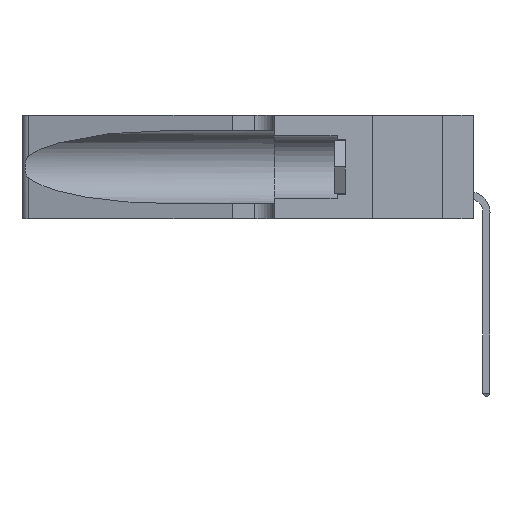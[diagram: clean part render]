
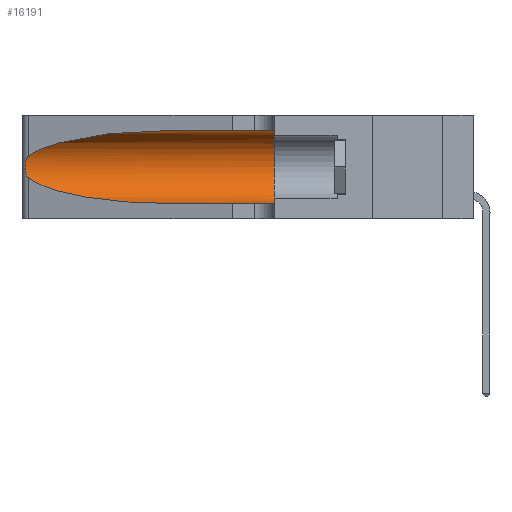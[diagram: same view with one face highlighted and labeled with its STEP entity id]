
A CAD part, left-side view. The second image highlights one B-rep face of the part: STEP entity #16191.
In plain terms, the highlighted cylindrical face has radius 3.308 mm (diameter 6.617 mm), a partial arc.
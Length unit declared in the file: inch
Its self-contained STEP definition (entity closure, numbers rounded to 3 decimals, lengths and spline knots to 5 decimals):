
#150 = VERTEX_POINT ( 'NONE', #843 ) ;
#653 = VERTEX_POINT ( 'NONE', #6501 ) ;
#745 = B_SPLINE_CURVE_WITH_KNOTS ( 'NONE', 3,
 ( #17289, #8688, #10274, #8830, #12127, #12191, #3586, #5343, #17432, #19124, #15380, #17130, #3381, #6819 ),
 .UNSPECIFIED., .F., .F.,
 ( 4, 2, 2, 2, 2, 2, 4 ),
 ( 0., 0.00027, 0.00053, 0.00107, 0.0016, 0.00187, 0.00214 ),
 .UNSPECIFIED. ) ;
#843 = CARTESIAN_POINT ( 'NONE',  ( 0.1305, 0.72297, 0.31525 ) ) ;
#1633 = CARTESIAN_POINT ( 'NONE',  ( 0.1305, 0.35, 0.31525 ) ) ;
#2723 = CARTESIAN_POINT ( 'NONE',  ( 0.25487, 1.22718, 0.14631 ) ) ;
#2830 = ORIENTED_EDGE ( 'NONE', *, *, #17265, .F. ) ;
#3282 = CARTESIAN_POINT ( 'NONE',  ( 0.1305, 0.72297, 0.05475 ) ) ;
#3381 = CARTESIAN_POINT ( 'NONE',  ( 0.25555, 1.22993, 0.14849 ) ) ;
#3586 = CARTESIAN_POINT ( 'NONE',  ( 0.26075, 1.23896, 0.19203 ) ) ;
#3943 = CARTESIAN_POINT ( 'NONE',  ( 0.1305, 0.35, 0.185 ) ) ;
#4028 = CIRCLE ( 'NONE', #14323, 0.13025 ) ;
#4514 =( BOUNDED_CURVE ( )  B_SPLINE_CURVE ( 3, ( #4868, #8597, #6722, #3282 ),
 .UNSPECIFIED., .F., .F. ) 
 B_SPLINE_CURVE_WITH_KNOTS ( ( 4, 4 ),
 ( 3.44316, 4.71239 ),
 .UNSPECIFIED. ) 
 CURVE ( )  GEOMETRIC_REPRESENTATION_ITEM ( )  RATIONAL_B_SPLINE_CURVE ( ( 1., 0.87, 0.87, 1. ) ) 
 REPRESENTATION_ITEM ( '' )  );
#4747 = CARTESIAN_POINT ( 'NONE',  ( 0.1305, 1.61858, 0.05475 ) ) ;
#4868 = CARTESIAN_POINT ( 'NONE',  ( 0.25487, 1.22718, 0.14631 ) ) ;
#4878 = EDGE_CURVE ( 'NONE', #653, #9045, #8433, .T. ) ;
#5343 = CARTESIAN_POINT ( 'NONE',  ( 0.26075, 1.23896, 0.178 ) ) ;
#5452 = DIRECTION ( 'NONE',  ( 0., 0., -1. ) ) ;
#5642 = EDGE_CURVE ( 'NONE', #150, #10348, #14591, .T. ) ;
#6501 = CARTESIAN_POINT ( 'NONE',  ( 0.1305, 0.72297, 0.05475 ) ) ;
#6722 = CARTESIAN_POINT ( 'NONE',  ( 0.18966, 0.96281, 0.05475 ) ) ;
#6819 = CARTESIAN_POINT ( 'NONE',  ( 0.25487, 1.22718, 0.14631 ) ) ;
#6820 = VECTOR ( 'NONE', #20263, 39.37008 ) ;
#7023 = CARTESIAN_POINT ( 'NONE',  ( 0.1305, 1.61858, 0.31525 ) ) ;
#7446 = EDGE_CURVE ( 'NONE', #10348, #16426, #745, .T. ) ;
#7447 = DIRECTION ( 'NONE',  ( 0., 0., 1. ) ) ;
#7451 = VERTEX_POINT ( 'NONE', #1633 ) ;
#8433 = LINE ( 'NONE', #4747, #6820 ) ;
#8597 = CARTESIAN_POINT ( 'NONE',  ( 0.2373, 1.15595, 0.08982 ) ) ;
#8688 = CARTESIAN_POINT ( 'NONE',  ( 0.25555, 1.22994, 0.2215 ) ) ;
#8807 = CARTESIAN_POINT ( 'NONE',  ( 0.1305, 0.72297, 0.31525 ) ) ;
#8830 = CARTESIAN_POINT ( 'NONE',  ( 0.25787, 1.23484, 0.2124 ) ) ;
#9045 = VERTEX_POINT ( 'NONE', #18593 ) ;
#9908 = EDGE_LOOP ( 'NONE', ( #13677, #14777, #13236, #13305, #10698, #2830 ) ) ;
#10274 = CARTESIAN_POINT ( 'NONE',  ( 0.25639, 1.23184, 0.21858 ) ) ;
#10318 = CARTESIAN_POINT ( 'NONE',  ( 0.18966, 0.96281, 0.31525 ) ) ;
#10348 = VERTEX_POINT ( 'NONE', #16599 ) ;
#10531 = CARTESIAN_POINT ( 'NONE',  ( 0.25487, 1.22718, 0.22369 ) ) ;
#10698 = ORIENTED_EDGE ( 'NONE', *, *, #10965, .F. ) ;
#10965 = EDGE_CURVE ( 'NONE', #7451, #9045, #4028, .T. ) ;
#12127 = CARTESIAN_POINT ( 'NONE',  ( 0.25854, 1.2359, 0.20912 ) ) ;
#12191 = CARTESIAN_POINT ( 'NONE',  ( 0.26018, 1.23835, 0.19895 ) ) ;
#13236 = ORIENTED_EDGE ( 'NONE', *, *, #14409, .T. ) ;
#13305 = ORIENTED_EDGE ( 'NONE', *, *, #4878, .T. ) ;
#13535 = AXIS2_PLACEMENT_3D ( 'NONE', #19157, #13953, #5452 ) ;
#13677 = ORIENTED_EDGE ( 'NONE', *, *, #5642, .T. ) ;
#13953 = DIRECTION ( 'NONE',  ( 0., -1., 0. ) ) ;
#14323 = AXIS2_PLACEMENT_3D ( 'NONE', #3943, #20861, #7447 ) ;
#14409 = EDGE_CURVE ( 'NONE', #16426, #653, #4514, .T. ) ;
#14591 =( BOUNDED_CURVE ( )  B_SPLINE_CURVE ( 3, ( #8807, #10318, #20790, #10531 ),
 .UNSPECIFIED., .F., .F. ) 
 B_SPLINE_CURVE_WITH_KNOTS ( ( 4, 4 ),
 ( 1.5708, 2.84003 ),
 .UNSPECIFIED. ) 
 CURVE ( )  GEOMETRIC_REPRESENTATION_ITEM ( )  RATIONAL_B_SPLINE_CURVE ( ( 1., 0.87, 0.87, 1. ) ) 
 REPRESENTATION_ITEM ( '' )  );
#14699 = LINE ( 'NONE', #7023, #15777 ) ;
#14722 = CYLINDRICAL_SURFACE ( 'NONE', #13535, 0.13025 ) ;
#14777 = ORIENTED_EDGE ( 'NONE', *, *, #7446, .T. ) ;
#15380 = CARTESIAN_POINT ( 'NONE',  ( 0.25789, 1.23486, 0.15765 ) ) ;
#15777 = VECTOR ( 'NONE', #18973, 39.37008 ) ;
#16191 = ADVANCED_FACE ( 'NONE', ( #18225 ), #14722, .F. ) ;
#16426 = VERTEX_POINT ( 'NONE', #2723 ) ;
#16599 = CARTESIAN_POINT ( 'NONE',  ( 0.25487, 1.22718, 0.22369 ) ) ;
#17130 = CARTESIAN_POINT ( 'NONE',  ( 0.25639, 1.23186, 0.15144 ) ) ;
#17265 = EDGE_CURVE ( 'NONE', #150, #7451, #14699, .T. ) ;
#17289 = CARTESIAN_POINT ( 'NONE',  ( 0.25487, 1.22718, 0.22369 ) ) ;
#17432 = CARTESIAN_POINT ( 'NONE',  ( 0.26017, 1.23833, 0.17102 ) ) ;
#18225 = FACE_OUTER_BOUND ( 'NONE', #9908, .T. ) ;
#18593 = CARTESIAN_POINT ( 'NONE',  ( 0.1305, 0.35, 0.05475 ) ) ;
#18973 = DIRECTION ( 'NONE',  ( 0., -1., 0. ) ) ;
#19124 = CARTESIAN_POINT ( 'NONE',  ( 0.25856, 1.23593, 0.16098 ) ) ;
#19157 = CARTESIAN_POINT ( 'NONE',  ( 0.1305, 1.61858, 0.185 ) ) ;
#20263 = DIRECTION ( 'NONE',  ( 0., -1., 0. ) ) ;
#20790 = CARTESIAN_POINT ( 'NONE',  ( 0.2373, 1.15595, 0.28018 ) ) ;
#20861 = DIRECTION ( 'NONE',  ( 0., 1., 0. ) ) ;
